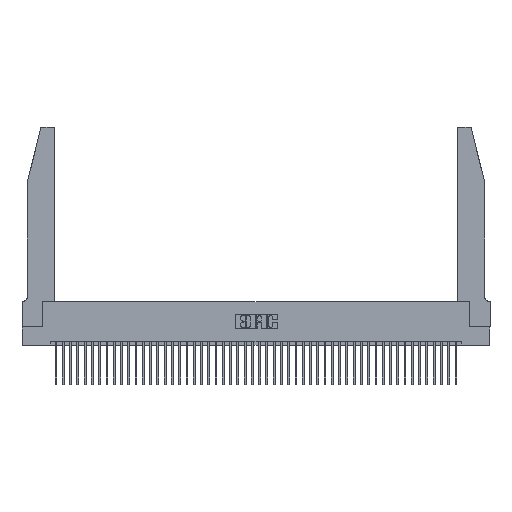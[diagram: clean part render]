
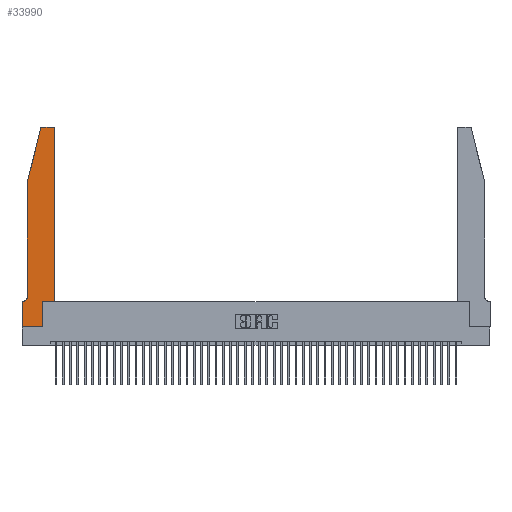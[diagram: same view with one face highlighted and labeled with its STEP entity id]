
A CAD part, top view. The second image highlights one B-rep face of the part: STEP entity #33990.
In plain terms, the highlighted planar face has unit normal (0, 0, 1).
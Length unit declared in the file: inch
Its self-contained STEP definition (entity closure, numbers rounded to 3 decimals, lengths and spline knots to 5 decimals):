
#260 = AXIS2_PLACEMENT_3D ( 'NONE', #14705, #7624, #32903 ) ;
#683 = VECTOR ( 'NONE', #9997, 39.37008 ) ;
#994 = CARTESIAN_POINT ( 'NONE',  ( 0.2605, 2.75, 0.37 ) ) ;
#1701 = VECTOR ( 'NONE', #38103, 39.37008 ) ;
#2092 = ORIENTED_EDGE ( 'NONE', *, *, #18106, .T. ) ;
#2493 = EDGE_CURVE ( 'NONE', #37347, #37684, #9138, .T. ) ;
#3085 = VECTOR ( 'NONE', #25224, 39.37008 ) ;
#3663 = CIRCLE ( 'NONE', #21631, 0.03 ) ;
#4965 = AXIS2_PLACEMENT_3D ( 'NONE', #37637, #15931, #41261 ) ;
#5183 = VERTEX_POINT ( 'NONE', #14496 ) ;
#6338 = ORIENTED_EDGE ( 'NONE', *, *, #11880, .T. ) ;
#6458 = DIRECTION ( 'NONE',  ( 0., 0., 1. ) ) ;
#6577 = VERTEX_POINT ( 'NONE', #30573 ) ;
#7312 = CARTESIAN_POINT ( 'NONE',  ( 0., 0., 0.37 ) ) ;
#7624 = DIRECTION ( 'NONE',  ( 0., 0., 1. ) ) ;
#8036 = DIRECTION ( 'NONE',  ( 1., 0., 0. ) ) ;
#8786 = EDGE_CURVE ( 'NONE', #37684, #36424, #43830, .T. ) ;
#9138 = LINE ( 'NONE', #13454, #683 ) ;
#9403 = LINE ( 'NONE', #33543, #15593 ) ;
#9541 = ORIENTED_EDGE ( 'NONE', *, *, #23341, .T. ) ;
#9716 = CARTESIAN_POINT ( 'NONE',  ( 0.0755, 0.42, 0.37 ) ) ;
#9997 = DIRECTION ( 'NONE',  ( 1., 0., 0. ) ) ;
#10122 = ORIENTED_EDGE ( 'NONE', *, *, #28326, .T. ) ;
#10567 = ORIENTED_EDGE ( 'NONE', *, *, #8786, .T. ) ;
#10699 = LINE ( 'NONE', #29697, #21462 ) ;
#10873 = CARTESIAN_POINT ( 'NONE',  ( 0.0755, 0.35, 0.37 ) ) ;
#11289 = LINE ( 'NONE', #45243, #1701 ) ;
#11880 = EDGE_CURVE ( 'NONE', #16398, #37347, #31924, .T. ) ;
#12707 = EDGE_CURVE ( 'NONE', #27107, #6577, #45551, .T. ) ;
#13454 = CARTESIAN_POINT ( 'NONE',  ( 0.4505, 0.35, 0.37 ) ) ;
#14416 = CARTESIAN_POINT ( 'NONE',  ( 0.0755, 2., 0.37 ) ) ;
#14496 = CARTESIAN_POINT ( 'NONE',  ( 0., 0.35, 0.37 ) ) ;
#14499 = VERTEX_POINT ( 'NONE', #9716 ) ;
#14579 = CARTESIAN_POINT ( 'NONE',  ( 0.4205, 2.72, 0.37 ) ) ;
#14705 = CARTESIAN_POINT ( 'NONE',  ( 0., 0.35, 0.37 ) ) ;
#15593 = VECTOR ( 'NONE', #37343, 39.37008 ) ;
#15931 = DIRECTION ( 'NONE',  ( 0., 0., -1. ) ) ;
#16038 = VECTOR ( 'NONE', #33572, 39.37008 ) ;
#16398 = VERTEX_POINT ( 'NONE', #17137 ) ;
#17017 = ORIENTED_EDGE ( 'NONE', *, *, #2493, .T. ) ;
#17137 = CARTESIAN_POINT ( 'NONE',  ( 0.2865, 0., 0.37 ) ) ;
#17928 = EDGE_CURVE ( 'NONE', #6577, #45174, #3663, .T. ) ;
#18037 = CARTESIAN_POINT ( 'NONE',  ( 0., 0., 0.37 ) ) ;
#18106 = EDGE_CURVE ( 'NONE', #41415, #5183, #41536, .T. ) ;
#18218 = DIRECTION ( 'NONE',  ( 1., 0., 0. ) ) ;
#19883 = CARTESIAN_POINT ( 'NONE',  ( 0.2865, 0.35, 0.37 ) ) ;
#21426 = VECTOR ( 'NONE', #36264, 39.37008 ) ;
#21462 = VECTOR ( 'NONE', #8036, 39.37008 ) ;
#21584 = CARTESIAN_POINT ( 'NONE',  ( 0.2865, 0.35, 0.37 ) ) ;
#21597 = CARTESIAN_POINT ( 'NONE',  ( 0.4505, 0.35, 0.37 ) ) ;
#21631 = AXIS2_PLACEMENT_3D ( 'NONE', #28113, #6458, #31745 ) ;
#23341 = EDGE_CURVE ( 'NONE', #5183, #40556, #41814, .T. ) ;
#25224 = DIRECTION ( 'NONE',  ( 0., 1., 0. ) ) ;
#25974 = ORIENTED_EDGE ( 'NONE', *, *, #12707, .T. ) ;
#26028 = CARTESIAN_POINT ( 'NONE',  ( 0.4205, 2.75, 0.37 ) ) ;
#26161 = ORIENTED_EDGE ( 'NONE', *, *, #17928, .T. ) ;
#26296 = CARTESIAN_POINT ( 'NONE',  ( 0.4505, 0.35, 0.37 ) ) ;
#27107 = VERTEX_POINT ( 'NONE', #26028 ) ;
#27237 = ORIENTED_EDGE ( 'NONE', *, *, #31435, .T. ) ;
#28113 = CARTESIAN_POINT ( 'NONE',  ( 0.284, 2.72, 0.37 ) ) ;
#28326 = EDGE_CURVE ( 'NONE', #14499, #41415, #35108, .T. ) ;
#28453 = EDGE_CURVE ( 'NONE', #44551, #14499, #11289, .T. ) ;
#28663 = CARTESIAN_POINT ( 'NONE',  ( 0.4505, 2.72, 0.37 ) ) ;
#28772 = CARTESIAN_POINT ( 'NONE',  ( 0.25487, 2.72718, 0.37 ) ) ;
#29464 = FACE_OUTER_BOUND ( 'NONE', #30507, .T. ) ;
#29697 = CARTESIAN_POINT ( 'NONE',  ( 0., 0., 0.37 ) ) ;
#29865 = ORIENTED_EDGE ( 'NONE', *, *, #28453, .T. ) ;
#30507 = EDGE_LOOP ( 'NONE', ( #25974, #26161, #46376, #29865, #10122, #2092, #9541, #30889, #6338, #17017, #10567, #27237 ) ) ;
#30573 = CARTESIAN_POINT ( 'NONE',  ( 0.284, 2.75, 0.37 ) ) ;
#30741 = CIRCLE ( 'NONE', #31679, 0.03 ) ;
#30889 = ORIENTED_EDGE ( 'NONE', *, *, #34703, .T. ) ;
#31435 = EDGE_CURVE ( 'NONE', #36424, #27107, #30741, .T. ) ;
#31679 = AXIS2_PLACEMENT_3D ( 'NONE', #14579, #39908, #18218 ) ;
#31745 = DIRECTION ( 'NONE',  ( 1., 0., 0. ) ) ;
#31918 = VECTOR ( 'NONE', #36195, 39.37008 ) ;
#31924 = LINE ( 'NONE', #21584, #3085 ) ;
#32903 = DIRECTION ( 'NONE',  ( 1., 0., 0. ) ) ;
#33543 = CARTESIAN_POINT ( 'NONE',  ( 0.0755, 2., 0.37 ) ) ;
#33572 = DIRECTION ( 'NONE',  ( 0., 1., 0. ) ) ;
#33990 = ADVANCED_FACE ( 'NONE', ( #29464 ), #43704, .T. ) ;
#34703 = EDGE_CURVE ( 'NONE', #40556, #16398, #10699, .T. ) ;
#35108 = CIRCLE ( 'NONE', #4965, 0.07 ) ;
#36195 = DIRECTION ( 'NONE',  ( -1., 0., 0. ) ) ;
#36264 = DIRECTION ( 'NONE',  ( 0., -1., 0. ) ) ;
#36424 = VERTEX_POINT ( 'NONE', #28663 ) ;
#37193 = DIRECTION ( 'NONE',  ( -1., 0., 0. ) ) ;
#37343 = DIRECTION ( 'NONE',  ( -0.239, -0.971, 0. ) ) ;
#37347 = VERTEX_POINT ( 'NONE', #19883 ) ;
#37637 = CARTESIAN_POINT ( 'NONE',  ( 0.0055, 0.42, 0.37 ) ) ;
#37684 = VERTEX_POINT ( 'NONE', #21597 ) ;
#38103 = DIRECTION ( 'NONE',  ( 0., -1., 0. ) ) ;
#39908 = DIRECTION ( 'NONE',  ( 0., 0., 1. ) ) ;
#40556 = VERTEX_POINT ( 'NONE', #7312 ) ;
#40745 = EDGE_CURVE ( 'NONE', #45174, #44551, #9403, .T. ) ;
#41261 = DIRECTION ( 'NONE',  ( -1., 0., 0. ) ) ;
#41415 = VERTEX_POINT ( 'NONE', #41437 ) ;
#41437 = CARTESIAN_POINT ( 'NONE',  ( 0.0055, 0.35, 0.37 ) ) ;
#41536 = LINE ( 'NONE', #10873, #31918 ) ;
#41814 = LINE ( 'NONE', #18037, #21426 ) ;
#43704 = PLANE ( 'NONE',  #260 ) ;
#43830 = LINE ( 'NONE', #26296, #16038 ) ;
#44423 = VECTOR ( 'NONE', #37193, 39.37008 ) ;
#44551 = VERTEX_POINT ( 'NONE', #14416 ) ;
#45174 = VERTEX_POINT ( 'NONE', #28772 ) ;
#45243 = CARTESIAN_POINT ( 'NONE',  ( 0.0755, 2., 0.37 ) ) ;
#45551 = LINE ( 'NONE', #994, #44423 ) ;
#46376 = ORIENTED_EDGE ( 'NONE', *, *, #40745, .T. ) ;
